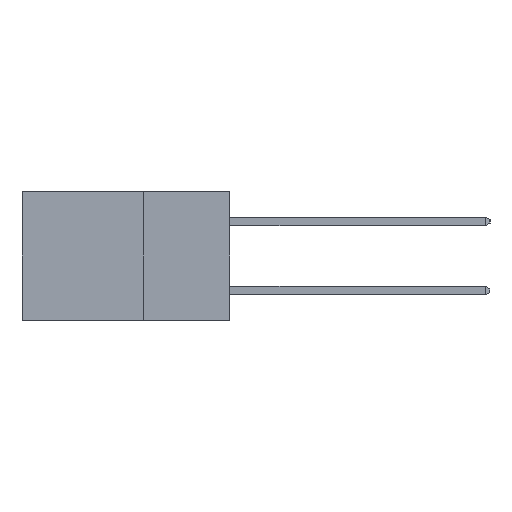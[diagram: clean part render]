
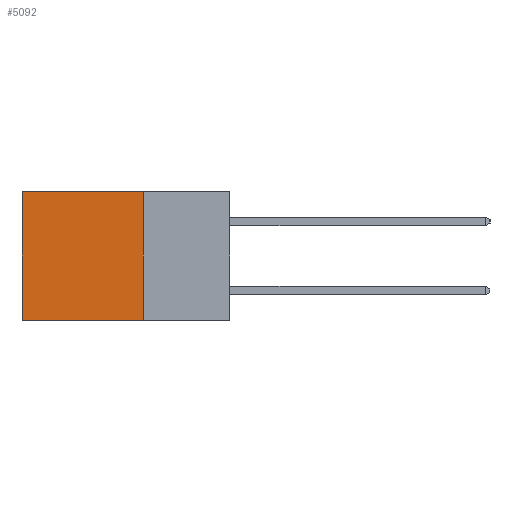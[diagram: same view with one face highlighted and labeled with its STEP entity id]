
A CAD part, left-side view. The second image highlights one B-rep face of the part: STEP entity #5092.
In plain terms, the highlighted planar face has unit normal (-1, 0, 0).
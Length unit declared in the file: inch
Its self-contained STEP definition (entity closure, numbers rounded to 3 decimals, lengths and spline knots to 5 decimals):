
#260 = CARTESIAN_POINT ( 'NONE',  ( 0.298, 0.25, 0. ) ) ;
#273 = EDGE_CURVE ( 'NONE', #3074, #2769, #559, .T. ) ;
#549 = LINE ( 'NONE', #3603, #8832 ) ;
#559 = LINE ( 'NONE', #2333, #12043 ) ;
#1058 = AXIS2_PLACEMENT_3D ( 'NONE', #6061, #2959, #2670 ) ;
#2187 = LINE ( 'NONE', #260, #4830 ) ;
#2333 = CARTESIAN_POINT ( 'NONE',  ( 0.298, 0.25, 0. ) ) ;
#2516 = ORIENTED_EDGE ( 'NONE', *, *, #12833, .T. ) ;
#2670 = DIRECTION ( 'NONE',  ( 0., 0., -1. ) ) ;
#2769 = VERTEX_POINT ( 'NONE', #2805 ) ;
#2805 = CARTESIAN_POINT ( 'NONE',  ( 0.298, 0.25, -0.37 ) ) ;
#2820 = DIRECTION ( 'NONE',  ( 0., 0., -1. ) ) ;
#2959 = DIRECTION ( 'NONE',  ( 1., 0., 0. ) ) ;
#3074 = VERTEX_POINT ( 'NONE', #5159 ) ;
#3399 = EDGE_LOOP ( 'NONE', ( #7205, #10986, #11386, #2516 ) ) ;
#3603 = CARTESIAN_POINT ( 'NONE',  ( 0.298, 0.25, -0.37 ) ) ;
#3708 = VERTEX_POINT ( 'NONE', #9957 ) ;
#3751 = DIRECTION ( 'NONE',  ( 0., 1., 0. ) ) ;
#4830 = VECTOR ( 'NONE', #3751, 39.37008 ) ;
#5092 = ADVANCED_FACE ( 'NONE', ( #9814 ), #11939, .F. ) ;
#5159 = CARTESIAN_POINT ( 'NONE',  ( 0.298, 0.25, 0. ) ) ;
#5651 = VECTOR ( 'NONE', #10490, 39.37008 ) ;
#6061 = CARTESIAN_POINT ( 'NONE',  ( 0.298, 0.25, 0. ) ) ;
#6501 = VERTEX_POINT ( 'NONE', #7699 ) ;
#7205 = ORIENTED_EDGE ( 'NONE', *, *, #7993, .T. ) ;
#7699 = CARTESIAN_POINT ( 'NONE',  ( 0.298, 0.6, 0. ) ) ;
#7993 = EDGE_CURVE ( 'NONE', #6501, #3708, #11175, .T. ) ;
#8832 = VECTOR ( 'NONE', #9130, 39.37008 ) ;
#9130 = DIRECTION ( 'NONE',  ( 0., 1., 0. ) ) ;
#9814 = FACE_OUTER_BOUND ( 'NONE', #3399, .T. ) ;
#9848 = CARTESIAN_POINT ( 'NONE',  ( 0.298, 0.6, 0. ) ) ;
#9957 = CARTESIAN_POINT ( 'NONE',  ( 0.298, 0.6, -0.37 ) ) ;
#10490 = DIRECTION ( 'NONE',  ( 0., 0., -1. ) ) ;
#10986 = ORIENTED_EDGE ( 'NONE', *, *, #12785, .F. ) ;
#11175 = LINE ( 'NONE', #9848, #5651 ) ;
#11386 = ORIENTED_EDGE ( 'NONE', *, *, #273, .F. ) ;
#11939 = PLANE ( 'NONE',  #1058 ) ;
#12043 = VECTOR ( 'NONE', #2820, 39.37008 ) ;
#12785 = EDGE_CURVE ( 'NONE', #2769, #3708, #549, .T. ) ;
#12833 = EDGE_CURVE ( 'NONE', #3074, #6501, #2187, .T. ) ;
